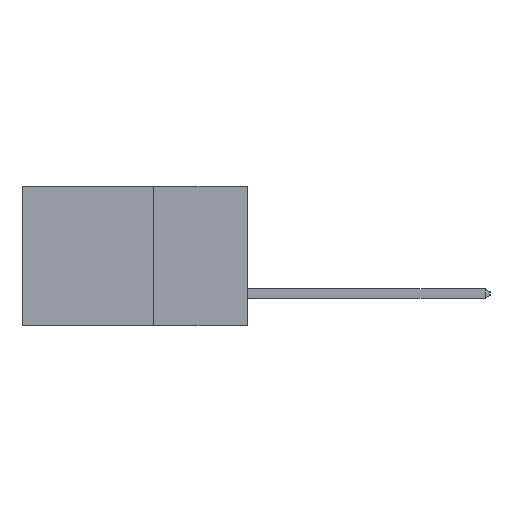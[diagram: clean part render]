
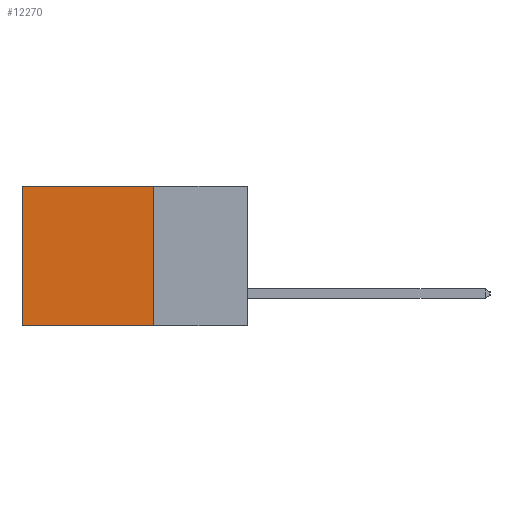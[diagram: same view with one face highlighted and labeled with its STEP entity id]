
A CAD part, left-side view. The second image highlights one B-rep face of the part: STEP entity #12270.
In plain terms, the highlighted planar face has unit normal (-1, 0, 0).
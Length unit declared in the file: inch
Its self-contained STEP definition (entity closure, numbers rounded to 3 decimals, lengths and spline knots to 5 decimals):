
#169 = DIRECTION ( 'NONE',  ( 0., 0., -1. ) ) ;
#858 = CARTESIAN_POINT ( 'NONE',  ( 0.298, 0.6, 0. ) ) ;
#1199 = CARTESIAN_POINT ( 'NONE',  ( 0.298, 0.25, 0. ) ) ;
#1233 = EDGE_CURVE ( 'NONE', #11177, #5202, #3171, .T. ) ;
#1332 = VECTOR ( 'NONE', #169, 39.37008 ) ;
#1771 = PLANE ( 'NONE',  #13880 ) ;
#2220 = LINE ( 'NONE', #2999, #4451 ) ;
#2889 = DIRECTION ( 'NONE',  ( 1., 0., 0. ) ) ;
#2951 = LINE ( 'NONE', #12519, #8746 ) ;
#2999 = CARTESIAN_POINT ( 'NONE',  ( 0.298, 0.25, 0. ) ) ;
#3171 = LINE ( 'NONE', #10384, #6085 ) ;
#3924 = LINE ( 'NONE', #13214, #1332 ) ;
#4451 = VECTOR ( 'NONE', #11692, 39.37008 ) ;
#4545 = VERTEX_POINT ( 'NONE', #858 ) ;
#5050 = DIRECTION ( 'NONE',  ( 0., 1., 0. ) ) ;
#5202 = VERTEX_POINT ( 'NONE', #11327 ) ;
#6085 = VECTOR ( 'NONE', #5050, 39.37008 ) ;
#6859 = FACE_OUTER_BOUND ( 'NONE', #9732, .T. ) ;
#8746 = VECTOR ( 'NONE', #13565, 39.37008 ) ;
#9173 = EDGE_CURVE ( 'NONE', #11428, #11177, #2951, .T. ) ;
#9409 = CARTESIAN_POINT ( 'NONE',  ( 0.298, 0.25, 0. ) ) ;
#9512 = CARTESIAN_POINT ( 'NONE',  ( 0.298, 0.25, -0.37 ) ) ;
#9732 = EDGE_LOOP ( 'NONE', ( #10555, #12780, #13496, #11464 ) ) ;
#10384 = CARTESIAN_POINT ( 'NONE',  ( 0.298, 0.25, -0.37 ) ) ;
#10486 = DIRECTION ( 'NONE',  ( 0., 0., -1. ) ) ;
#10555 = ORIENTED_EDGE ( 'NONE', *, *, #13182, .T. ) ;
#11177 = VERTEX_POINT ( 'NONE', #9512 ) ;
#11195 = EDGE_CURVE ( 'NONE', #11428, #4545, #2220, .T. ) ;
#11327 = CARTESIAN_POINT ( 'NONE',  ( 0.298, 0.6, -0.37 ) ) ;
#11428 = VERTEX_POINT ( 'NONE', #1199 ) ;
#11464 = ORIENTED_EDGE ( 'NONE', *, *, #11195, .T. ) ;
#11692 = DIRECTION ( 'NONE',  ( 0., 1., 0. ) ) ;
#12270 = ADVANCED_FACE ( 'NONE', ( #6859 ), #1771, .F. ) ;
#12519 = CARTESIAN_POINT ( 'NONE',  ( 0.298, 0.25, 0. ) ) ;
#12780 = ORIENTED_EDGE ( 'NONE', *, *, #1233, .F. ) ;
#13182 = EDGE_CURVE ( 'NONE', #4545, #5202, #3924, .T. ) ;
#13214 = CARTESIAN_POINT ( 'NONE',  ( 0.298, 0.6, 0. ) ) ;
#13496 = ORIENTED_EDGE ( 'NONE', *, *, #9173, .F. ) ;
#13565 = DIRECTION ( 'NONE',  ( 0., 0., -1. ) ) ;
#13880 = AXIS2_PLACEMENT_3D ( 'NONE', #9409, #2889, #10486 ) ;
